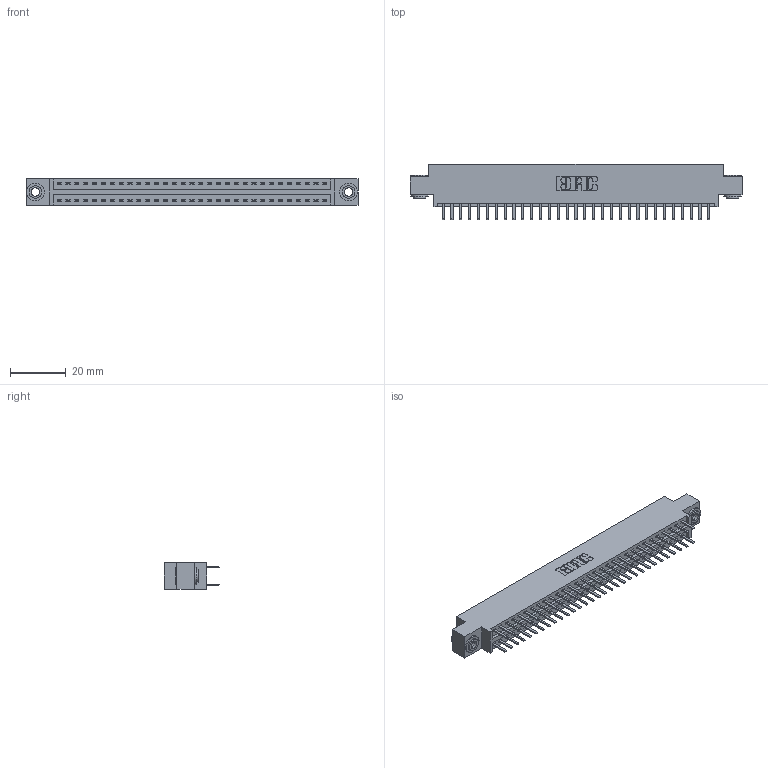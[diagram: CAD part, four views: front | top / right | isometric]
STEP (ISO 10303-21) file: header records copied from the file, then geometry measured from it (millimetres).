
FILE_DESCRIPTION (( 'STEP AP203' ), '1' );
FILE_NAME ('346-062-520-803.STEP', '2022-05-24T13:17:47', ( '' ), ( '' ), 'SwSTEP 2.0', 'SolidWorks 2020', '' );
FILE_SCHEMA (( 'CONFIG_CONTROL_DESIGN' ));
Length unit declared in the file: inch
Products named in the file (4): 346 Part_0.170 Offset - 0.156 Dia-TH; 345-292-001_345-293-120; 345-250-002_345-250-002-102; 346-062-520-803
Assembly tree (65 placements, depth 2):
  346-062-520-803
    346 Part_0.170 Offset - 0.156 Dia-TH
    345-292-001_345-293-120  x62
    345-250-002_345-250-002-102  x2
Bounding box: 119 x 20.02 x 9.4 mm (x, y, z)
Volume: 11337.9 mm3; surface area: 15776.3 mm2
Topology: 65 solids, 65 shells, 3650 faces, 10559 edges, 6870 vertices
Faces by surface type: plane 2398, cylinder 1244, cone 8
Entity records: 23024 total; most frequent: CARTESIAN_POINT 3805, ORIENTED_EDGE 3718, DIRECTION 3421, EDGE_CURVE 1859, LINE 1575, VECTOR 1575, VERTEX_POINT 1234, AXIS2_PLACEMENT_3D 923
